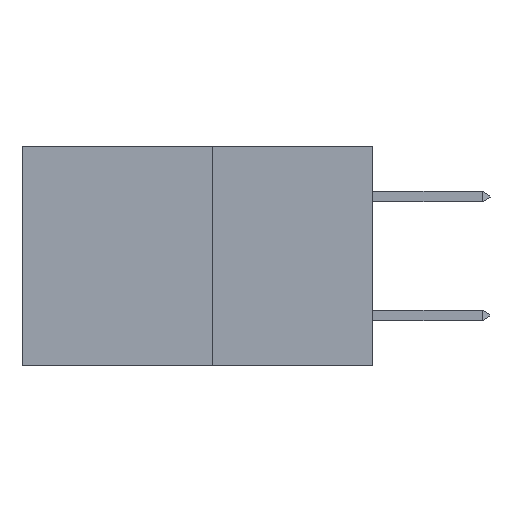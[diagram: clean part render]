
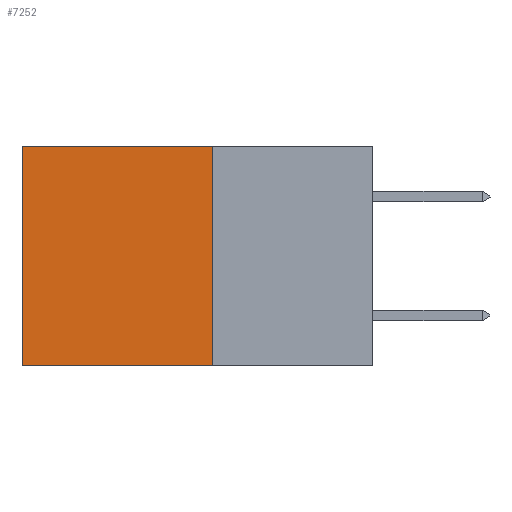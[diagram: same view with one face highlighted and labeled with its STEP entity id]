
A CAD part, left-side view. The second image highlights one B-rep face of the part: STEP entity #7252.
In plain terms, the highlighted planar face has unit normal (-1, 0, 0).
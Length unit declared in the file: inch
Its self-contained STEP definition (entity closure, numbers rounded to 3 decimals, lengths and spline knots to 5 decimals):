
#80 = VERTEX_POINT ( 'NONE', #1479 ) ;
#264 = ORIENTED_EDGE ( 'NONE', *, *, #3532, .F. ) ;
#351 = EDGE_CURVE ( 'NONE', #80, #761, #4702, .T. ) ;
#648 = CARTESIAN_POINT ( 'NONE',  ( 0.277, 0.27, -0.37 ) ) ;
#761 = VERTEX_POINT ( 'NONE', #966 ) ;
#863 = DIRECTION ( 'NONE',  ( 0., 1., 0. ) ) ;
#966 = CARTESIAN_POINT ( 'NONE',  ( 0.277, 0.59, 0. ) ) ;
#1053 = DIRECTION ( 'NONE',  ( 0., 0., -1. ) ) ;
#1479 = CARTESIAN_POINT ( 'NONE',  ( 0.277, 0.27, 0. ) ) ;
#1614 = CARTESIAN_POINT ( 'NONE',  ( 0.277, 0.27, -0.37 ) ) ;
#2371 = VECTOR ( 'NONE', #4379, 39.37008 ) ;
#2886 = EDGE_CURVE ( 'NONE', #80, #8299, #6261, .T. ) ;
#2989 = FACE_OUTER_BOUND ( 'NONE', #8049, .T. ) ;
#3005 = LINE ( 'NONE', #7301, #8425 ) ;
#3455 = DIRECTION ( 'NONE',  ( 1., 0., 0. ) ) ;
#3487 = ORIENTED_EDGE ( 'NONE', *, *, #2886, .F. ) ;
#3532 = EDGE_CURVE ( 'NONE', #8299, #6396, #5726, .T. ) ;
#3650 = DIRECTION ( 'NONE',  ( 0., 0., -1. ) ) ;
#4379 = DIRECTION ( 'NONE',  ( 0., 0., -1. ) ) ;
#4444 = ORIENTED_EDGE ( 'NONE', *, *, #6387, .T. ) ;
#4580 = CARTESIAN_POINT ( 'NONE',  ( 0.277, 0.27, 0. ) ) ;
#4702 = LINE ( 'NONE', #4580, #6516 ) ;
#5047 = PLANE ( 'NONE',  #7348 ) ;
#5379 = CARTESIAN_POINT ( 'NONE',  ( 0.277, 0.27, -0.37 ) ) ;
#5726 = LINE ( 'NONE', #648, #7281 ) ;
#5859 = ORIENTED_EDGE ( 'NONE', *, *, #351, .T. ) ;
#6261 = LINE ( 'NONE', #5379, #2371 ) ;
#6387 = EDGE_CURVE ( 'NONE', #761, #6396, #3005, .T. ) ;
#6396 = VERTEX_POINT ( 'NONE', #8844 ) ;
#6516 = VECTOR ( 'NONE', #863, 39.37008 ) ;
#7243 = CARTESIAN_POINT ( 'NONE',  ( 0.277, 0.27, -0.37 ) ) ;
#7252 = ADVANCED_FACE ( 'NONE', ( #2989 ), #5047, .F. ) ;
#7281 = VECTOR ( 'NONE', #7423, 39.37008 ) ;
#7301 = CARTESIAN_POINT ( 'NONE',  ( 0.277, 0.59, -0.37 ) ) ;
#7348 = AXIS2_PLACEMENT_3D ( 'NONE', #1614, #3455, #1053 ) ;
#7423 = DIRECTION ( 'NONE',  ( 0., 1., 0. ) ) ;
#8049 = EDGE_LOOP ( 'NONE', ( #4444, #264, #3487, #5859 ) ) ;
#8299 = VERTEX_POINT ( 'NONE', #7243 ) ;
#8425 = VECTOR ( 'NONE', #3650, 39.37008 ) ;
#8844 = CARTESIAN_POINT ( 'NONE',  ( 0.277, 0.59, -0.37 ) ) ;
